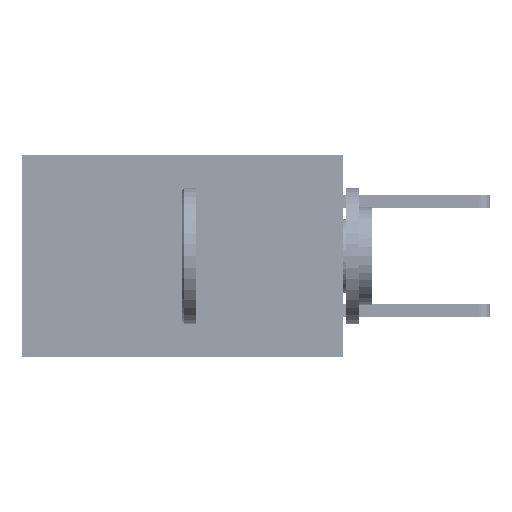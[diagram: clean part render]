
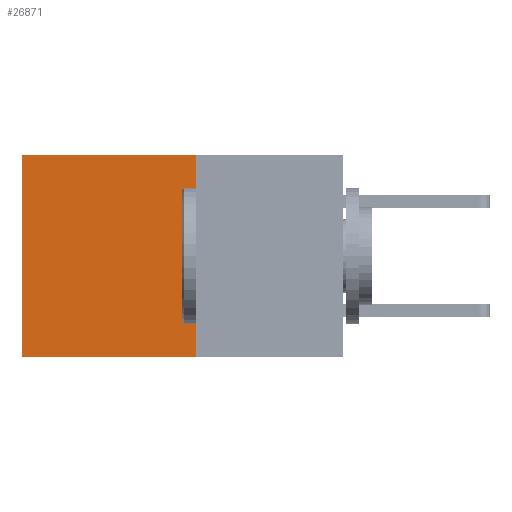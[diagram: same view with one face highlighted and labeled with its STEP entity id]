
A CAD part, left-side view. The second image highlights one B-rep face of the part: STEP entity #26871.
In plain terms, the highlighted planar face has unit normal (-1, 0, 0).
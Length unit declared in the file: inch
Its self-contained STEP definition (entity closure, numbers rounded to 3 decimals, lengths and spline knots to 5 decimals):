
#167 = ORIENTED_EDGE ( 'NONE', *, *, #23190, .T. ) ;
#771 = CARTESIAN_POINT ( 'NONE',  ( 0.277, 0.27, 0. ) ) ;
#3393 = ORIENTED_EDGE ( 'NONE', *, *, #8944, .F. ) ;
#4041 = CARTESIAN_POINT ( 'NONE',  ( 0.277, 0.27, -0.37 ) ) ;
#4999 = VERTEX_POINT ( 'NONE', #17790 ) ;
#5174 = FACE_OUTER_BOUND ( 'NONE', #34868, .T. ) ;
#5549 = EDGE_CURVE ( 'NONE', #4999, #12893, #6323, .T. ) ;
#6323 = LINE ( 'NONE', #771, #25741 ) ;
#7834 = VECTOR ( 'NONE', #25537, 39.37008 ) ;
#8944 = EDGE_CURVE ( 'NONE', #24474, #27350, #28456, .T. ) ;
#9929 = CARTESIAN_POINT ( 'NONE',  ( 0.277, 0.59, -0.37 ) ) ;
#11432 = EDGE_CURVE ( 'NONE', #4999, #24474, #31142, .T. ) ;
#11712 = DIRECTION ( 'NONE',  ( 0., 0., -1. ) ) ;
#12893 = VERTEX_POINT ( 'NONE', #34343 ) ;
#14664 = CARTESIAN_POINT ( 'NONE',  ( 0.277, 0.59, -0.37 ) ) ;
#17790 = CARTESIAN_POINT ( 'NONE',  ( 0.277, 0.27, 0. ) ) ;
#18523 = DIRECTION ( 'NONE',  ( 0., 0., -1. ) ) ;
#18894 = ORIENTED_EDGE ( 'NONE', *, *, #11432, .F. ) ;
#19496 = DIRECTION ( 'NONE',  ( 0., 1., 0. ) ) ;
#21187 = CARTESIAN_POINT ( 'NONE',  ( 0.277, 0.27, -0.37 ) ) ;
#21324 = VECTOR ( 'NONE', #11712, 39.37008 ) ;
#21572 = AXIS2_PLACEMENT_3D ( 'NONE', #21187, #32082, #18523 ) ;
#23083 = DIRECTION ( 'NONE',  ( 0., 1., 0. ) ) ;
#23190 = EDGE_CURVE ( 'NONE', #12893, #27350, #24823, .T. ) ;
#24474 = VERTEX_POINT ( 'NONE', #29176 ) ;
#24651 = VECTOR ( 'NONE', #23083, 39.37008 ) ;
#24823 = LINE ( 'NONE', #14664, #7834 ) ;
#25537 = DIRECTION ( 'NONE',  ( 0., 0., -1. ) ) ;
#25741 = VECTOR ( 'NONE', #19496, 39.37008 ) ;
#26871 = ADVANCED_FACE ( 'NONE', ( #5174 ), #29773, .F. ) ;
#27350 = VERTEX_POINT ( 'NONE', #9929 ) ;
#28275 = ORIENTED_EDGE ( 'NONE', *, *, #5549, .T. ) ;
#28456 = LINE ( 'NONE', #4041, #24651 ) ;
#29176 = CARTESIAN_POINT ( 'NONE',  ( 0.277, 0.27, -0.37 ) ) ;
#29773 = PLANE ( 'NONE',  #21572 ) ;
#31142 = LINE ( 'NONE', #33992, #21324 ) ;
#32082 = DIRECTION ( 'NONE',  ( 1., 0., 0. ) ) ;
#33992 = CARTESIAN_POINT ( 'NONE',  ( 0.277, 0.27, -0.37 ) ) ;
#34343 = CARTESIAN_POINT ( 'NONE',  ( 0.277, 0.59, 0. ) ) ;
#34868 = EDGE_LOOP ( 'NONE', ( #167, #3393, #18894, #28275 ) ) ;
